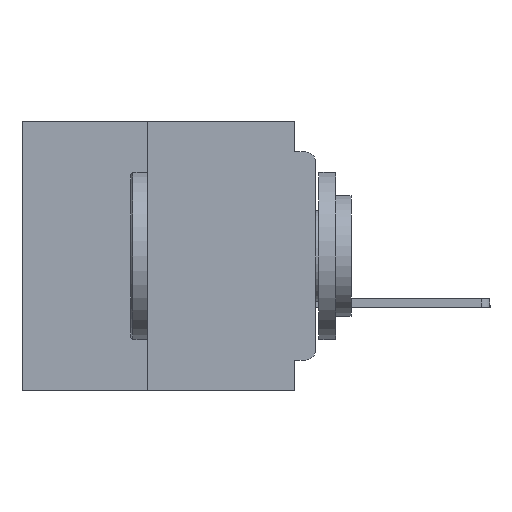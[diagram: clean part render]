
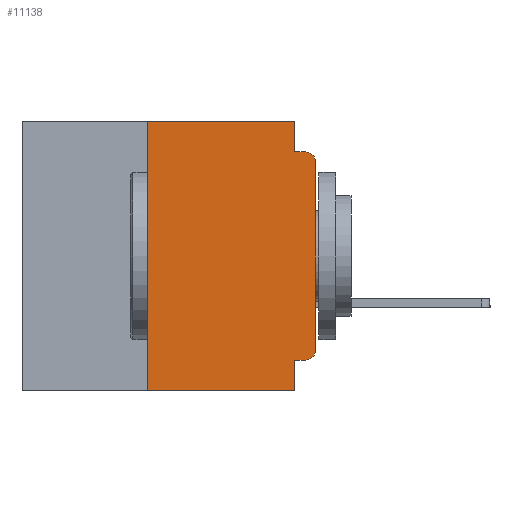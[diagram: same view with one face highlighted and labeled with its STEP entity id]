
A CAD part, left-side view. The second image highlights one B-rep face of the part: STEP entity #11138.
In plain terms, the highlighted planar face has unit normal (-1, 0, 0).
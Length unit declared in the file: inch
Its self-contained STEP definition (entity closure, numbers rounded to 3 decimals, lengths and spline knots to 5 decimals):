
#26 = EDGE_CURVE ( 'NONE', #5886, #4618, #38469, .T. ) ;
#209 = CARTESIAN_POINT ( 'NONE',  ( 0., 0.015, -0.06 ) ) ;
#2241 = ORIENTED_EDGE ( 'NONE', *, *, #9450, .T. ) ;
#2808 = DIRECTION ( 'NONE',  ( 0., -1., 0. ) ) ;
#2865 = ORIENTED_EDGE ( 'NONE', *, *, #25681, .F. ) ;
#3082 = VECTOR ( 'NONE', #26671, 39.37008 ) ;
#3439 = VECTOR ( 'NONE', #4995, 39.37008 ) ;
#4189 = DIRECTION ( 'NONE',  ( 0., 0., -1. ) ) ;
#4367 = VERTEX_POINT ( 'NONE', #32975 ) ;
#4618 = VERTEX_POINT ( 'NONE', #46118 ) ;
#4881 = CARTESIAN_POINT ( 'NONE',  ( 0., 0.015, -0.045 ) ) ;
#4995 = DIRECTION ( 'NONE',  ( 0., -1., 0. ) ) ;
#5076 = CIRCLE ( 'NONE', #48741, 0.015 ) ;
#5129 = VECTOR ( 'NONE', #22754, 39.37008 ) ;
#5385 = VERTEX_POINT ( 'NONE', #29852 ) ;
#5761 = DIRECTION ( 'NONE',  ( -1., 0., 0. ) ) ;
#5779 = VECTOR ( 'NONE', #13274, 39.37008 ) ;
#5886 = VERTEX_POINT ( 'NONE', #48573 ) ;
#6569 = CARTESIAN_POINT ( 'NONE',  ( 0., 0.031, -0.4 ) ) ;
#9148 = EDGE_CURVE ( 'NONE', #47223, #16765, #36932, .T. ) ;
#9450 = EDGE_CURVE ( 'NONE', #16344, #38859, #27141, .T. ) ;
#11138 = ADVANCED_FACE ( 'NONE', ( #33658 ), #33773, .F. ) ;
#12449 = ORIENTED_EDGE ( 'NONE', *, *, #26, .F. ) ;
#12560 = CARTESIAN_POINT ( 'NONE',  ( 0., 0.25, -0.4 ) ) ;
#13274 = DIRECTION ( 'NONE',  ( 0., -1., 0. ) ) ;
#13564 = LINE ( 'NONE', #34519, #3082 ) ;
#14354 = DIRECTION ( 'NONE',  ( 0., 0., -1. ) ) ;
#15084 = VERTEX_POINT ( 'NONE', #4881 ) ;
#15874 = ORIENTED_EDGE ( 'NONE', *, *, #29453, .F. ) ;
#16344 = VERTEX_POINT ( 'NONE', #23515 ) ;
#16496 = DIRECTION ( 'NONE',  ( 0., 0., 1. ) ) ;
#16765 = VERTEX_POINT ( 'NONE', #6569 ) ;
#17286 = DIRECTION ( 'NONE',  ( 0., 0., -1. ) ) ;
#20320 = ORIENTED_EDGE ( 'NONE', *, *, #34944, .T. ) ;
#20721 = ORIENTED_EDGE ( 'NONE', *, *, #43510, .F. ) ;
#21093 = CARTESIAN_POINT ( 'NONE',  ( 0., 0.437, -0.4 ) ) ;
#22453 = CARTESIAN_POINT ( 'NONE',  ( 0., 0.25, -0.4 ) ) ;
#22754 = DIRECTION ( 'NONE',  ( 0., 0., 1. ) ) ;
#23113 = LINE ( 'NONE', #12560, #31041 ) ;
#23385 = DIRECTION ( 'NONE',  ( 0., 1., 0. ) ) ;
#23515 = CARTESIAN_POINT ( 'NONE',  ( 0., 0., -0.34 ) ) ;
#24283 = VERTEX_POINT ( 'NONE', #30890 ) ;
#25507 = LINE ( 'NONE', #43822, #3439 ) ;
#25681 = EDGE_CURVE ( 'NONE', #5385, #24283, #25908, .T. ) ;
#25908 = LINE ( 'NONE', #36735, #36262 ) ;
#26671 = DIRECTION ( 'NONE',  ( 0., 0., -1. ) ) ;
#27141 = LINE ( 'NONE', #49906, #5129 ) ;
#27600 = DIRECTION ( 'NONE',  ( -1., 0., 0. ) ) ;
#28136 = VECTOR ( 'NONE', #23385, 39.37008 ) ;
#28516 = ORIENTED_EDGE ( 'NONE', *, *, #45811, .F. ) ;
#29174 = CARTESIAN_POINT ( 'NONE',  ( 0., 0.015, -0.34 ) ) ;
#29217 = ORIENTED_EDGE ( 'NONE', *, *, #36967, .F. ) ;
#29453 = EDGE_CURVE ( 'NONE', #47223, #4367, #23113, .T. ) ;
#29852 = CARTESIAN_POINT ( 'NONE',  ( 0., 0.031, 0. ) ) ;
#30890 = CARTESIAN_POINT ( 'NONE',  ( 0., 0.031, -0.045 ) ) ;
#31041 = VECTOR ( 'NONE', #16496, 39.37008 ) ;
#32643 = AXIS2_PLACEMENT_3D ( 'NONE', #29174, #5761, #33081 ) ;
#32975 = CARTESIAN_POINT ( 'NONE',  ( 0., 0.25, 0. ) ) ;
#33081 = DIRECTION ( 'NONE',  ( 0., 0., -1. ) ) ;
#33658 = FACE_OUTER_BOUND ( 'NONE', #36797, .T. ) ;
#33773 = PLANE ( 'NONE',  #34294 ) ;
#34026 = ORIENTED_EDGE ( 'NONE', *, *, #40494, .T. ) ;
#34294 = AXIS2_PLACEMENT_3D ( 'NONE', #49145, #37668, #14354 ) ;
#34519 = CARTESIAN_POINT ( 'NONE',  ( 0., 0.031, -0.4 ) ) ;
#34944 = EDGE_CURVE ( 'NONE', #5886, #16344, #35815, .T. ) ;
#34985 = LINE ( 'NONE', #49470, #42829 ) ;
#35815 = CIRCLE ( 'NONE', #32643, 0.015 ) ;
#36262 = VECTOR ( 'NONE', #17286, 39.37008 ) ;
#36735 = CARTESIAN_POINT ( 'NONE',  ( 0., 0.031, 0. ) ) ;
#36792 = CARTESIAN_POINT ( 'NONE',  ( 0., 0., -0.06 ) ) ;
#36797 = EDGE_LOOP ( 'NONE', ( #2241, #34026, #29217, #2865, #28516, #15874, #37876, #20721, #12449, #20320 ) ) ;
#36932 = LINE ( 'NONE', #21093, #5779 ) ;
#36967 = EDGE_CURVE ( 'NONE', #24283, #15084, #34985, .T. ) ;
#37668 = DIRECTION ( 'NONE',  ( 1., 0., 0. ) ) ;
#37876 = ORIENTED_EDGE ( 'NONE', *, *, #9148, .T. ) ;
#38469 = LINE ( 'NONE', #39372, #28136 ) ;
#38859 = VERTEX_POINT ( 'NONE', #36792 ) ;
#39372 = CARTESIAN_POINT ( 'NONE',  ( 0., 0., -0.355 ) ) ;
#40494 = EDGE_CURVE ( 'NONE', #38859, #15084, #5076, .T. ) ;
#42829 = VECTOR ( 'NONE', #2808, 39.37008 ) ;
#43510 = EDGE_CURVE ( 'NONE', #4618, #16765, #13564, .T. ) ;
#43822 = CARTESIAN_POINT ( 'NONE',  ( 0., 0.437, 0. ) ) ;
#45811 = EDGE_CURVE ( 'NONE', #4367, #5385, #25507, .T. ) ;
#46118 = CARTESIAN_POINT ( 'NONE',  ( 0., 0.031, -0.355 ) ) ;
#47223 = VERTEX_POINT ( 'NONE', #22453 ) ;
#48573 = CARTESIAN_POINT ( 'NONE',  ( 0., 0.015, -0.355 ) ) ;
#48741 = AXIS2_PLACEMENT_3D ( 'NONE', #209, #27600, #4189 ) ;
#49145 = CARTESIAN_POINT ( 'NONE',  ( 0., 0.437, 0. ) ) ;
#49470 = CARTESIAN_POINT ( 'NONE',  ( 0., 0., -0.045 ) ) ;
#49906 = CARTESIAN_POINT ( 'NONE',  ( 0., 0., 0. ) ) ;
